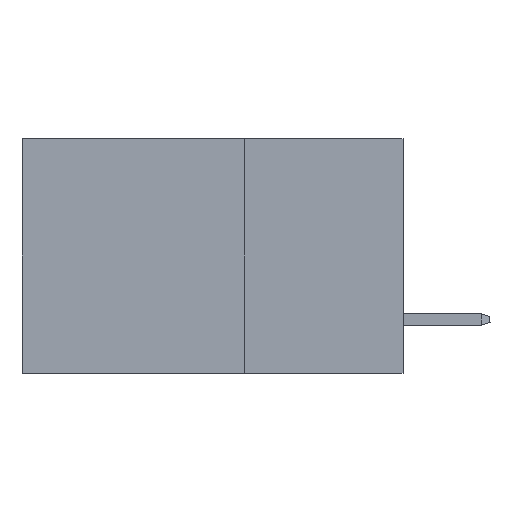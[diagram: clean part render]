
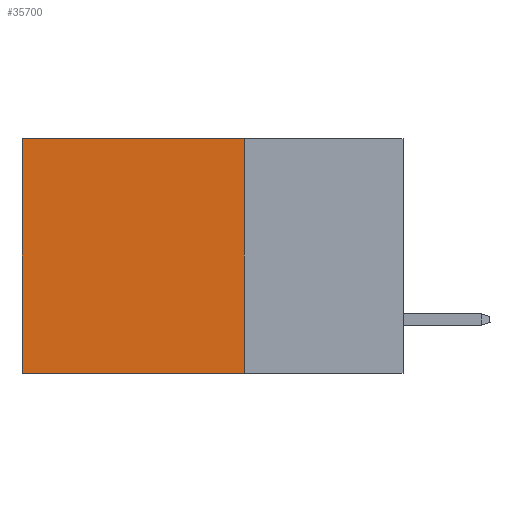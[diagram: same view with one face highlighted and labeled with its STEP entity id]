
A CAD part, left-side view. The second image highlights one B-rep face of the part: STEP entity #35700.
In plain terms, the highlighted planar face has unit normal (-1, 0, 0).
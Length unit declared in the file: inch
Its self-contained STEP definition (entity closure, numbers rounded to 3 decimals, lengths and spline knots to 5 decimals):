
#441 = FACE_OUTER_BOUND ( 'NONE', #8613, .T. ) ;
#499 = VECTOR ( 'NONE', #36506, 39.37008 ) ;
#573 = LINE ( 'NONE', #3639, #36838 ) ;
#767 = ORIENTED_EDGE ( 'NONE', *, *, #4181, .F. ) ;
#1981 = VERTEX_POINT ( 'NONE', #16757 ) ;
#3174 = CARTESIAN_POINT ( 'NONE',  ( 0.2875, 0.6, -0.37 ) ) ;
#3420 = EDGE_CURVE ( 'NONE', #36700, #1981, #30173, .T. ) ;
#3639 = CARTESIAN_POINT ( 'NONE',  ( 0.2875, 0.25, 0. ) ) ;
#4181 = EDGE_CURVE ( 'NONE', #4679, #15406, #36358, .T. ) ;
#4679 = VERTEX_POINT ( 'NONE', #14670 ) ;
#6772 = DIRECTION ( 'NONE',  ( 0., 0., -1. ) ) ;
#8613 = EDGE_LOOP ( 'NONE', ( #35587, #767, #18767, #38749 ) ) ;
#9407 = EDGE_CURVE ( 'NONE', #1981, #15406, #16395, .T. ) ;
#9547 = DIRECTION ( 'NONE',  ( 0., 0., -1. ) ) ;
#10327 = VECTOR ( 'NONE', #20449, 39.37008 ) ;
#12898 = CARTESIAN_POINT ( 'NONE',  ( 0.2875, 0.25, 0. ) ) ;
#13101 = CARTESIAN_POINT ( 'NONE',  ( 0.2875, 0.6, 0. ) ) ;
#14670 = CARTESIAN_POINT ( 'NONE',  ( 0.2875, 0.25, -0.37 ) ) ;
#15406 = VERTEX_POINT ( 'NONE', #3174 ) ;
#16250 = VECTOR ( 'NONE', #38623, 39.37008 ) ;
#16395 = LINE ( 'NONE', #13101, #16250 ) ;
#16698 = CARTESIAN_POINT ( 'NONE',  ( 0.2875, 0.25, 0. ) ) ;
#16757 = CARTESIAN_POINT ( 'NONE',  ( 0.2875, 0.6, 0. ) ) ;
#18767 = ORIENTED_EDGE ( 'NONE', *, *, #25163, .F. ) ;
#20449 = DIRECTION ( 'NONE',  ( 0., 1., 0. ) ) ;
#22118 = PLANE ( 'NONE',  #29450 ) ;
#24085 = CARTESIAN_POINT ( 'NONE',  ( 0.2875, 0.25, 0. ) ) ;
#25163 = EDGE_CURVE ( 'NONE', #36700, #4679, #573, .T. ) ;
#29450 = AXIS2_PLACEMENT_3D ( 'NONE', #12898, #31286, #6772 ) ;
#30173 = LINE ( 'NONE', #24085, #499 ) ;
#30645 = CARTESIAN_POINT ( 'NONE',  ( 0.2875, 0.25, -0.37 ) ) ;
#31286 = DIRECTION ( 'NONE',  ( 1., 0., 0. ) ) ;
#35587 = ORIENTED_EDGE ( 'NONE', *, *, #9407, .T. ) ;
#35700 = ADVANCED_FACE ( 'NONE', ( #441 ), #22118, .F. ) ;
#36358 = LINE ( 'NONE', #30645, #10327 ) ;
#36506 = DIRECTION ( 'NONE',  ( 0., 1., 0. ) ) ;
#36700 = VERTEX_POINT ( 'NONE', #16698 ) ;
#36838 = VECTOR ( 'NONE', #9547, 39.37008 ) ;
#38623 = DIRECTION ( 'NONE',  ( 0., 0., -1. ) ) ;
#38749 = ORIENTED_EDGE ( 'NONE', *, *, #3420, .T. ) ;
